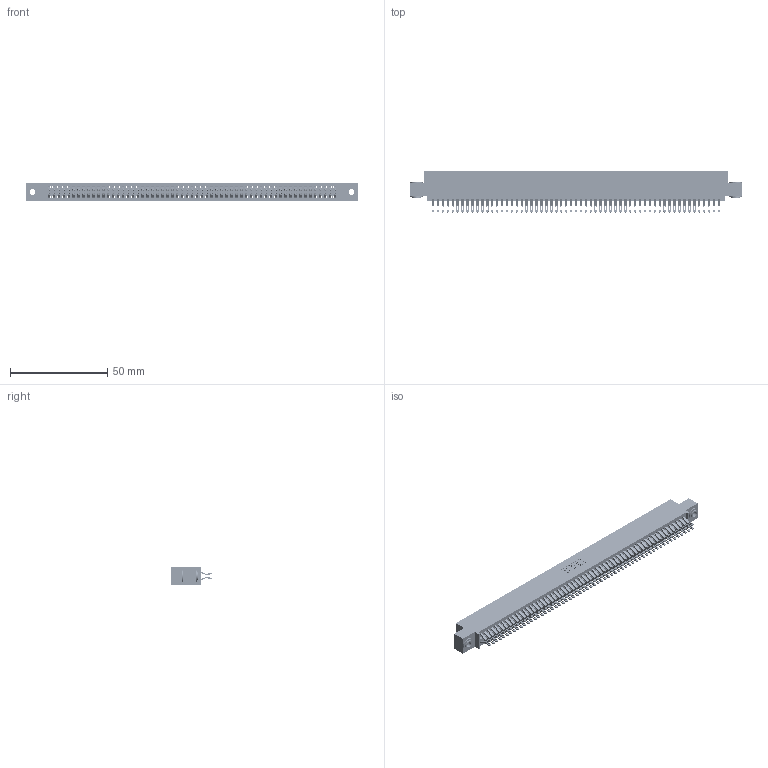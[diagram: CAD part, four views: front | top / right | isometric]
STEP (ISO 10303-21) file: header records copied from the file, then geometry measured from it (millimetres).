
FILE_DESCRIPTION (( 'STEP AP203' ), '1' );
FILE_NAME ('345-118-555-503.STEP', '2019-11-05T21:20:08', ( '' ), ( '' ), 'SwSTEP 2.0', 'SolidWorks 2016', '' );
FILE_SCHEMA (( 'CONFIG_CONTROL_DESIGN' ));
Length unit declared in the file: inch
Products named in the file (4): 345-250-002_345-250-002-102; 345 Part_0.110 Offset - 0.156 Dia-TH; 345-292-001_555 Tail; 345-118-555-503
Assembly tree (121 placements, depth 2):
  345-118-555-503
    345 Part_0.110 Offset - 0.156 Dia-TH
    345-292-001_555 Tail  x118
    345-250-002_345-250-002-102  x2
Bounding box: 171.07 x 21.13 x 9.4 mm (x, y, z)
Volume: 17063.9 mm3; surface area: 27040.7 mm2
Topology: 121 solids, 121 shells, 6776 faces, 21315 edges, 14206 vertices
Faces by surface type: plane 3752, cylinder 3016, cone 8
Entity records: 45112 total; most frequent: CARTESIAN_POINT 7557, ORIENTED_EDGE 7454, DIRECTION 6641, EDGE_CURVE 3727, LINE 3315, VECTOR 3315, VERTEX_POINT 2482, AXIS2_PLACEMENT_3D 1663
